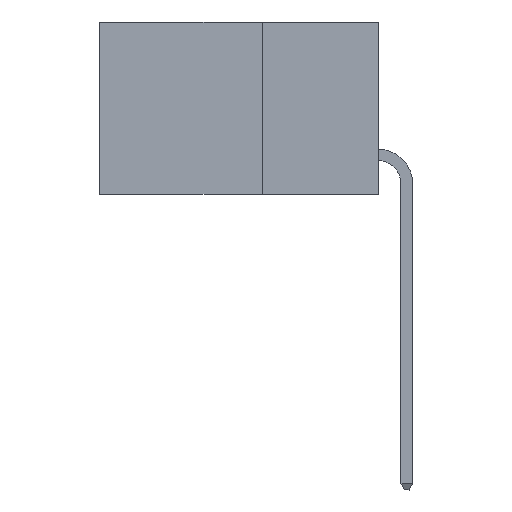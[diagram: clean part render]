
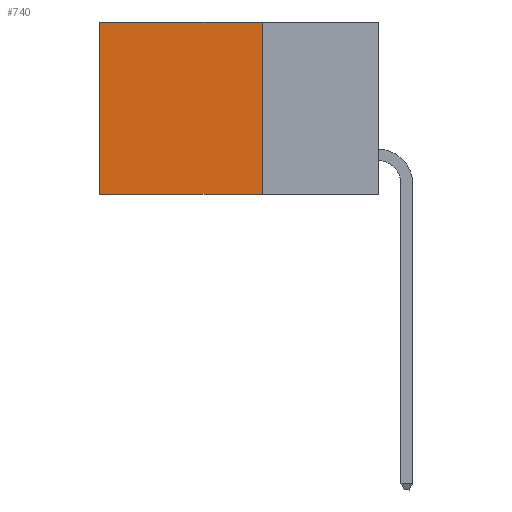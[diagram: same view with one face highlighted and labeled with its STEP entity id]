
A CAD part, left-side view. The second image highlights one B-rep face of the part: STEP entity #740.
In plain terms, the highlighted planar face has unit normal (-1, 0, 0).
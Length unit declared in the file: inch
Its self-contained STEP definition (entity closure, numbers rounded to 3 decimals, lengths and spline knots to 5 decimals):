
#579 = DIRECTION ( 'NONE',  ( 0., 1., 0. ) ) ;
#740 = ADVANCED_FACE ( 'NONE', ( #22743 ), #10804, .F. ) ;
#1180 = CARTESIAN_POINT ( 'NONE',  ( 0.298, 0.25, 0. ) ) ;
#2117 = LINE ( 'NONE', #1180, #13350 ) ;
#3261 = DIRECTION ( 'NONE',  ( 0., 0., -1. ) ) ;
#3411 = DIRECTION ( 'NONE',  ( 1., 0., 0. ) ) ;
#3651 = DIRECTION ( 'NONE',  ( 0., 0., -1. ) ) ;
#3704 = EDGE_CURVE ( 'NONE', #21694, #15639, #22005, .T. ) ;
#3876 = CARTESIAN_POINT ( 'NONE',  ( 0.298, 0.25, -0.37 ) ) ;
#4868 = LINE ( 'NONE', #7055, #16649 ) ;
#5737 = ORIENTED_EDGE ( 'NONE', *, *, #9425, .T. ) ;
#5745 = CARTESIAN_POINT ( 'NONE',  ( 0.298, 0.6, 0. ) ) ;
#6311 = VERTEX_POINT ( 'NONE', #3876 ) ;
#6435 = VERTEX_POINT ( 'NONE', #6721 ) ;
#6721 = CARTESIAN_POINT ( 'NONE',  ( 0.298, 0.6, -0.37 ) ) ;
#7055 = CARTESIAN_POINT ( 'NONE',  ( 0.298, 0.25, -0.37 ) ) ;
#7100 = CARTESIAN_POINT ( 'NONE',  ( 0.298, 0.6, 0. ) ) ;
#8303 = CARTESIAN_POINT ( 'NONE',  ( 0.298, 0.25, 0. ) ) ;
#9425 = EDGE_CURVE ( 'NONE', #15639, #6435, #12180, .T. ) ;
#10058 = EDGE_LOOP ( 'NONE', ( #5737, #14993, #13777, #16910 ) ) ;
#10804 = PLANE ( 'NONE',  #20037 ) ;
#12180 = LINE ( 'NONE', #7100, #20886 ) ;
#12314 = DIRECTION ( 'NONE',  ( 0., 1., 0. ) ) ;
#13350 = VECTOR ( 'NONE', #17225, 39.37008 ) ;
#13777 = ORIENTED_EDGE ( 'NONE', *, *, #17089, .F. ) ;
#14993 = ORIENTED_EDGE ( 'NONE', *, *, #22939, .F. ) ;
#15639 = VERTEX_POINT ( 'NONE', #5745 ) ;
#16649 = VECTOR ( 'NONE', #12314, 39.37008 ) ;
#16910 = ORIENTED_EDGE ( 'NONE', *, *, #3704, .T. ) ;
#16914 = CARTESIAN_POINT ( 'NONE',  ( 0.298, 0.25, 0. ) ) ;
#17089 = EDGE_CURVE ( 'NONE', #21694, #6311, #2117, .T. ) ;
#17225 = DIRECTION ( 'NONE',  ( 0., 0., -1. ) ) ;
#17228 = VECTOR ( 'NONE', #579, 39.37008 ) ;
#20037 = AXIS2_PLACEMENT_3D ( 'NONE', #21523, #3411, #3651 ) ;
#20886 = VECTOR ( 'NONE', #3261, 39.37008 ) ;
#21523 = CARTESIAN_POINT ( 'NONE',  ( 0.298, 0.25, 0. ) ) ;
#21694 = VERTEX_POINT ( 'NONE', #8303 ) ;
#22005 = LINE ( 'NONE', #16914, #17228 ) ;
#22743 = FACE_OUTER_BOUND ( 'NONE', #10058, .T. ) ;
#22939 = EDGE_CURVE ( 'NONE', #6311, #6435, #4868, .T. ) ;
